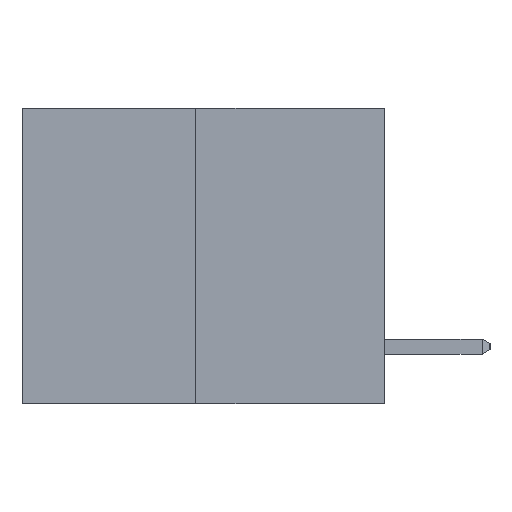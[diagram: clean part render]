
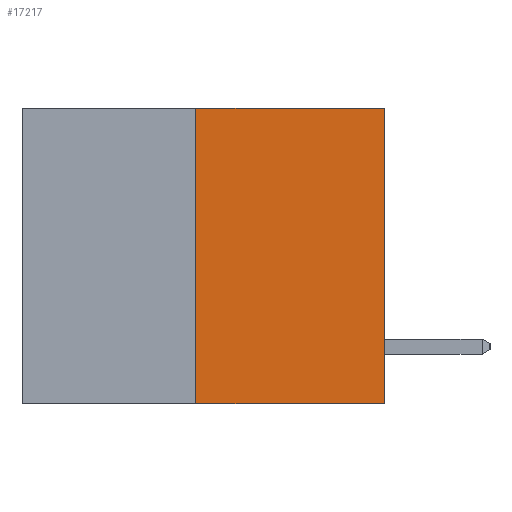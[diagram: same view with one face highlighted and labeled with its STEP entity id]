
A CAD part, left-side view. The second image highlights one B-rep face of the part: STEP entity #17217.
In plain terms, the highlighted planar face has unit normal (-1, 0, 0).
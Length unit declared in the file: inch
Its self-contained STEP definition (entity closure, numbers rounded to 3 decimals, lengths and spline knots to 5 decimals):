
#806 = LINE ( 'NONE', #21437, #14409 ) ;
#1850 = ORIENTED_EDGE ( 'NONE', *, *, #9906, .T. ) ;
#2087 = CARTESIAN_POINT ( 'NONE',  ( 0., 0., 0. ) ) ;
#2338 = FACE_OUTER_BOUND ( 'NONE', #10978, .T. ) ;
#3364 = DIRECTION ( 'NONE',  ( 0., 0., 1. ) ) ;
#3549 = DIRECTION ( 'NONE',  ( 0., 0., 1. ) ) ;
#4133 = EDGE_CURVE ( 'NONE', #9755, #15058, #14761, .T. ) ;
#4147 = VERTEX_POINT ( 'NONE', #11812 ) ;
#4594 = LINE ( 'NONE', #2087, #14016 ) ;
#4890 = CARTESIAN_POINT ( 'NONE',  ( 0., 0.312, -0.49 ) ) ;
#6703 = CARTESIAN_POINT ( 'NONE',  ( 0., 0.6, 0. ) ) ;
#7129 = CARTESIAN_POINT ( 'NONE',  ( 0., 0., 0. ) ) ;
#8570 = VERTEX_POINT ( 'NONE', #4890 ) ;
#9538 = PLANE ( 'NONE',  #18339 ) ;
#9755 = VERTEX_POINT ( 'NONE', #14241 ) ;
#9906 = EDGE_CURVE ( 'NONE', #8570, #4147, #16943, .T. ) ;
#10956 = ORIENTED_EDGE ( 'NONE', *, *, #11215, .T. ) ;
#10978 = EDGE_LOOP ( 'NONE', ( #18462, #1850, #10956, #19893 ) ) ;
#11215 = EDGE_CURVE ( 'NONE', #4147, #15058, #4594, .T. ) ;
#11812 = CARTESIAN_POINT ( 'NONE',  ( 0., 0., -0.49 ) ) ;
#12425 = VECTOR ( 'NONE', #14951, 39.37008 ) ;
#14016 = VECTOR ( 'NONE', #3549, 39.37008 ) ;
#14241 = CARTESIAN_POINT ( 'NONE',  ( 0., 0.312, 0. ) ) ;
#14409 = VECTOR ( 'NONE', #3364, 39.37008 ) ;
#14761 = LINE ( 'NONE', #6703, #12425 ) ;
#14951 = DIRECTION ( 'NONE',  ( 0., -1., 0. ) ) ;
#15058 = VERTEX_POINT ( 'NONE', #7129 ) ;
#16192 = CARTESIAN_POINT ( 'NONE',  ( 0., 0.6, 0. ) ) ;
#16765 = EDGE_CURVE ( 'NONE', #8570, #9755, #806, .T. ) ;
#16943 = LINE ( 'NONE', #20952, #20861 ) ;
#17217 = ADVANCED_FACE ( 'NONE', ( #2338 ), #9538, .F. ) ;
#17694 = DIRECTION ( 'NONE',  ( 0., -1., 0. ) ) ;
#18013 = DIRECTION ( 'NONE',  ( 1., 0., 0. ) ) ;
#18339 = AXIS2_PLACEMENT_3D ( 'NONE', #16192, #18013, #21345 ) ;
#18462 = ORIENTED_EDGE ( 'NONE', *, *, #16765, .F. ) ;
#19893 = ORIENTED_EDGE ( 'NONE', *, *, #4133, .F. ) ;
#20861 = VECTOR ( 'NONE', #17694, 39.37008 ) ;
#20952 = CARTESIAN_POINT ( 'NONE',  ( 0., 0.6, -0.49 ) ) ;
#21345 = DIRECTION ( 'NONE',  ( 0., 0., -1. ) ) ;
#21437 = CARTESIAN_POINT ( 'NONE',  ( 0., 0.312, -0.49 ) ) ;
